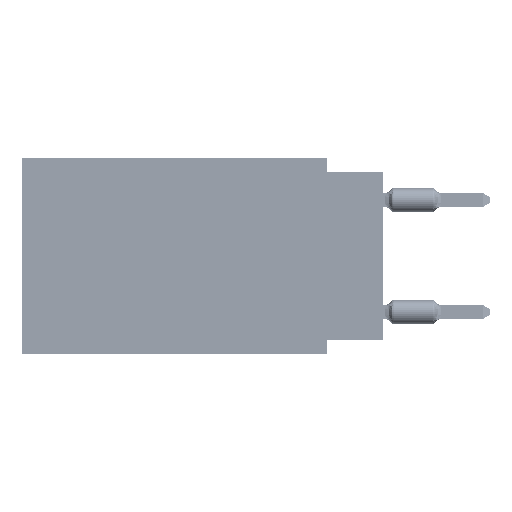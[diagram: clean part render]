
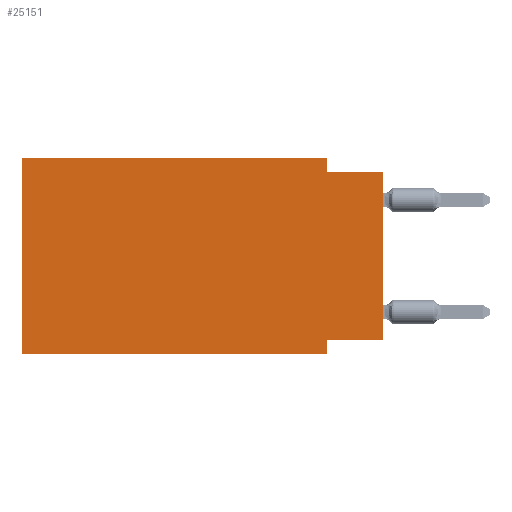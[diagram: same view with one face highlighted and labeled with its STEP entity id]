
A CAD part, left-side view. The second image highlights one B-rep face of the part: STEP entity #25151.
In plain terms, the highlighted planar face has unit normal (-1, 0, 0).
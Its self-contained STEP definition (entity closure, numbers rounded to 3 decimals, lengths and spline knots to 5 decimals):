
#8671 = LINE ( 'NONE', #27363, #99164 ) ;
#8960 = LINE ( 'NONE', #89612, #105245 ) ;
#9644 = VECTOR ( 'NONE', #18741, 39.37008 ) ;
#13502 = ORIENTED_EDGE ( 'NONE', *, *, #61360, .F. ) ;
#14616 = AXIS2_PLACEMENT_3D ( 'NONE', #23152, #85678, #69271 ) ;
#16083 = VERTEX_POINT ( 'NONE', #54792 ) ;
#16966 = CARTESIAN_POINT ( 'NONE',  ( 0., 0.1, -0.025 ) ) ;
#18741 = DIRECTION ( 'NONE',  ( 0., 1., 0. ) ) ;
#22495 = ORIENTED_EDGE ( 'NONE', *, *, #56010, .F. ) ;
#22500 = VECTOR ( 'NONE', #75727, 39.37008 ) ;
#23152 = CARTESIAN_POINT ( 'NONE',  ( 0., 0.645, 0. ) ) ;
#23701 = PLANE ( 'NONE',  #14616 ) ;
#25151 = ADVANCED_FACE ( 'NONE', ( #104372 ), #23701, .F. ) ;
#27363 = CARTESIAN_POINT ( 'NONE',  ( 0., 0., 0. ) ) ;
#28000 = VERTEX_POINT ( 'NONE', #31500 ) ;
#30362 = VERTEX_POINT ( 'NONE', #107701 ) ;
#31500 = CARTESIAN_POINT ( 'NONE',  ( 0., 0.645, -0.35 ) ) ;
#32750 = ORIENTED_EDGE ( 'NONE', *, *, #54486, .F. ) ;
#35718 = LINE ( 'NONE', #108192, #9644 ) ;
#38522 = LINE ( 'NONE', #109839, #96564 ) ;
#44557 = VERTEX_POINT ( 'NONE', #16966 ) ;
#44624 = DIRECTION ( 'NONE',  ( 0., -1., 0. ) ) ;
#46633 = VERTEX_POINT ( 'NONE', #73293 ) ;
#48757 = EDGE_CURVE ( 'NONE', #28000, #83173, #38522, .T. ) ;
#52854 = CARTESIAN_POINT ( 'NONE',  ( 0., 0.645, 0. ) ) ;
#53586 = EDGE_CURVE ( 'NONE', #30362, #83869, #8671, .T. ) ;
#54486 = EDGE_CURVE ( 'NONE', #30362, #16083, #35718, .T. ) ;
#54792 = CARTESIAN_POINT ( 'NONE',  ( 0., 0.1, -0.325 ) ) ;
#56010 = EDGE_CURVE ( 'NONE', #83173, #81931, #110676, .T. ) ;
#56287 = VECTOR ( 'NONE', #83750, 39.37008 ) ;
#56823 = CARTESIAN_POINT ( 'NONE',  ( 0., 0.1, 0. ) ) ;
#57204 = ORIENTED_EDGE ( 'NONE', *, *, #79664, .F. ) ;
#59332 = LINE ( 'NONE', #93861, #22500 ) ;
#61360 = EDGE_CURVE ( 'NONE', #81931, #44557, #64996, .T. ) ;
#62880 = ORIENTED_EDGE ( 'NONE', *, *, #53586, .T. ) ;
#63067 = DIRECTION ( 'NONE',  ( 0., 0., -1. ) ) ;
#64977 = ORIENTED_EDGE ( 'NONE', *, *, #87681, .T. ) ;
#64996 = LINE ( 'NONE', #56823, #88947 ) ;
#69271 = DIRECTION ( 'NONE',  ( 0., 0., -1. ) ) ;
#72442 = DIRECTION ( 'NONE',  ( 0., 0., 1. ) ) ;
#73293 = CARTESIAN_POINT ( 'NONE',  ( 0., 0.1, -0.35 ) ) ;
#75727 = DIRECTION ( 'NONE',  ( 0., -1., 0. ) ) ;
#79664 = EDGE_CURVE ( 'NONE', #16083, #46633, #81175, .T. ) ;
#81002 = ORIENTED_EDGE ( 'NONE', *, *, #48757, .F. ) ;
#81175 = LINE ( 'NONE', #100452, #114815 ) ;
#81931 = VERTEX_POINT ( 'NONE', #97819 ) ;
#83173 = VERTEX_POINT ( 'NONE', #52854 ) ;
#83750 = DIRECTION ( 'NONE',  ( 0., -1., 0. ) ) ;
#83869 = VERTEX_POINT ( 'NONE', #113387 ) ;
#85678 = DIRECTION ( 'NONE',  ( 1., 0., 0. ) ) ;
#86039 = CARTESIAN_POINT ( 'NONE',  ( 0., 0.645, 0. ) ) ;
#87681 = EDGE_CURVE ( 'NONE', #28000, #46633, #59332, .T. ) ;
#88947 = VECTOR ( 'NONE', #100657, 39.37008 ) ;
#89612 = CARTESIAN_POINT ( 'NONE',  ( 0., 0., -0.025 ) ) ;
#93861 = CARTESIAN_POINT ( 'NONE',  ( 0., 0.645, -0.35 ) ) ;
#96346 = DIRECTION ( 'NONE',  ( 0., 0., 1. ) ) ;
#96564 = VECTOR ( 'NONE', #72442, 39.37008 ) ;
#97819 = CARTESIAN_POINT ( 'NONE',  ( 0., 0.1, 0. ) ) ;
#99164 = VECTOR ( 'NONE', #96346, 39.37008 ) ;
#100452 = CARTESIAN_POINT ( 'NONE',  ( 0., 0.1, -0.35 ) ) ;
#100657 = DIRECTION ( 'NONE',  ( 0., 0., -1. ) ) ;
#102457 = ORIENTED_EDGE ( 'NONE', *, *, #111404, .F. ) ;
#104372 = FACE_OUTER_BOUND ( 'NONE', #110289, .T. ) ;
#105245 = VECTOR ( 'NONE', #44624, 39.37008 ) ;
#107701 = CARTESIAN_POINT ( 'NONE',  ( 0., 0., -0.325 ) ) ;
#108192 = CARTESIAN_POINT ( 'NONE',  ( 0., 0., -0.325 ) ) ;
#109839 = CARTESIAN_POINT ( 'NONE',  ( 0., 0.645, 0. ) ) ;
#110289 = EDGE_LOOP ( 'NONE', ( #62880, #102457, #13502, #22495, #81002, #64977, #57204, #32750 ) ) ;
#110676 = LINE ( 'NONE', #86039, #56287 ) ;
#111404 = EDGE_CURVE ( 'NONE', #44557, #83869, #8960, .T. ) ;
#113387 = CARTESIAN_POINT ( 'NONE',  ( 0., 0., -0.025 ) ) ;
#114815 = VECTOR ( 'NONE', #63067, 39.37008 ) ;
